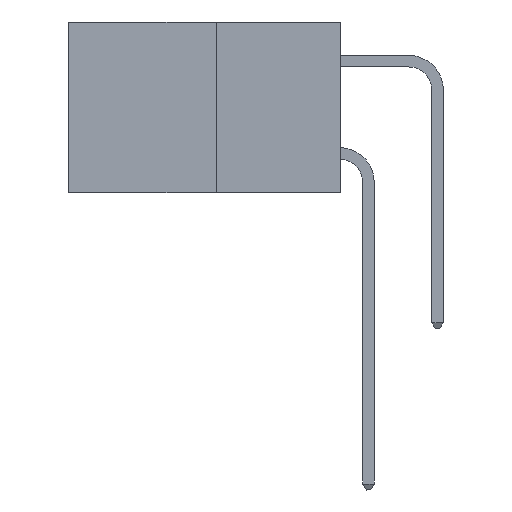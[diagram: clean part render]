
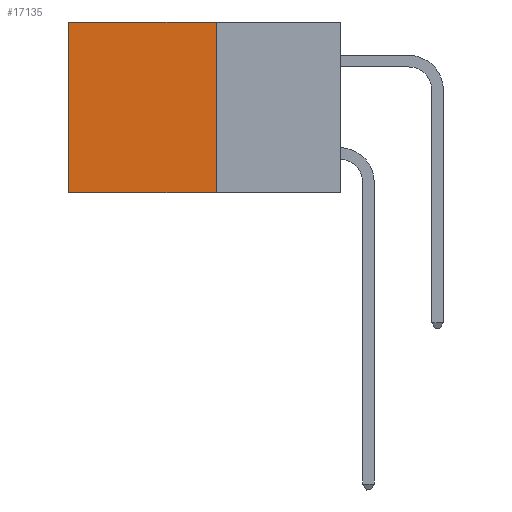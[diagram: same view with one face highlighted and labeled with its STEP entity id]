
A CAD part, left-side view. The second image highlights one B-rep face of the part: STEP entity #17135.
In plain terms, the highlighted planar face has unit normal (-1, 0, 0).
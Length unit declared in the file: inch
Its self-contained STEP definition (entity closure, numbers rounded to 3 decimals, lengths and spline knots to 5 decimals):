
#486 = CARTESIAN_POINT ( 'NONE',  ( 0.277, 0.59, -0.37 ) ) ;
#961 = CARTESIAN_POINT ( 'NONE',  ( 0.277, 0.27, -0.37 ) ) ;
#1854 = CARTESIAN_POINT ( 'NONE',  ( 0.277, 0.27, 0. ) ) ;
#2395 = VERTEX_POINT ( 'NONE', #1854 ) ;
#3217 = VECTOR ( 'NONE', #9747, 39.37008 ) ;
#3855 = LINE ( 'NONE', #8213, #6664 ) ;
#3943 = ORIENTED_EDGE ( 'NONE', *, *, #4655, .F. ) ;
#4037 = ORIENTED_EDGE ( 'NONE', *, *, #4607, .F. ) ;
#4607 = EDGE_CURVE ( 'NONE', #2395, #7861, #6086, .T. ) ;
#4655 = EDGE_CURVE ( 'NONE', #7861, #12052, #12455, .T. ) ;
#4809 = ORIENTED_EDGE ( 'NONE', *, *, #7521, .T. ) ;
#5135 = AXIS2_PLACEMENT_3D ( 'NONE', #6646, #15948, #8055 ) ;
#6086 = LINE ( 'NONE', #13799, #9327 ) ;
#6646 = CARTESIAN_POINT ( 'NONE',  ( 0.277, 0.27, -0.37 ) ) ;
#6664 = VECTOR ( 'NONE', #8743, 39.37008 ) ;
#6893 = LINE ( 'NONE', #14889, #3217 ) ;
#7146 = ORIENTED_EDGE ( 'NONE', *, *, #14983, .T. ) ;
#7521 = EDGE_CURVE ( 'NONE', #2395, #9101, #3855, .T. ) ;
#7861 = VERTEX_POINT ( 'NONE', #11746 ) ;
#8055 = DIRECTION ( 'NONE',  ( 0., 0., -1. ) ) ;
#8213 = CARTESIAN_POINT ( 'NONE',  ( 0.277, 0.27, 0. ) ) ;
#8463 = VECTOR ( 'NONE', #8564, 39.37008 ) ;
#8564 = DIRECTION ( 'NONE',  ( 0., 1., 0. ) ) ;
#8743 = DIRECTION ( 'NONE',  ( 0., 1., 0. ) ) ;
#9101 = VERTEX_POINT ( 'NONE', #13001 ) ;
#9173 = EDGE_LOOP ( 'NONE', ( #7146, #3943, #4037, #4809 ) ) ;
#9327 = VECTOR ( 'NONE', #14825, 39.37008 ) ;
#9747 = DIRECTION ( 'NONE',  ( 0., 0., -1. ) ) ;
#10275 = FACE_OUTER_BOUND ( 'NONE', #9173, .T. ) ;
#10731 = PLANE ( 'NONE',  #5135 ) ;
#11746 = CARTESIAN_POINT ( 'NONE',  ( 0.277, 0.27, -0.37 ) ) ;
#12052 = VERTEX_POINT ( 'NONE', #486 ) ;
#12455 = LINE ( 'NONE', #961, #8463 ) ;
#13001 = CARTESIAN_POINT ( 'NONE',  ( 0.277, 0.59, 0. ) ) ;
#13799 = CARTESIAN_POINT ( 'NONE',  ( 0.277, 0.27, -0.37 ) ) ;
#14825 = DIRECTION ( 'NONE',  ( 0., 0., -1. ) ) ;
#14889 = CARTESIAN_POINT ( 'NONE',  ( 0.277, 0.59, -0.37 ) ) ;
#14983 = EDGE_CURVE ( 'NONE', #9101, #12052, #6893, .T. ) ;
#15948 = DIRECTION ( 'NONE',  ( 1., 0., 0. ) ) ;
#17135 = ADVANCED_FACE ( 'NONE', ( #10275 ), #10731, .F. ) ;
